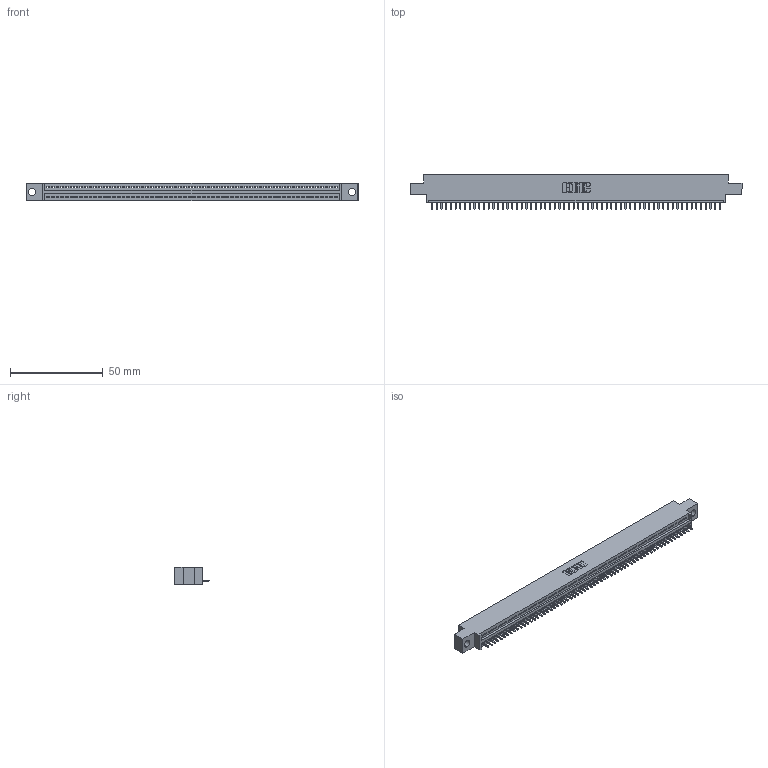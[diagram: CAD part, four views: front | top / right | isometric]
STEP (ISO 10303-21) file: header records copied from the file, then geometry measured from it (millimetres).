
FILE_DESCRIPTION (( 'STEP AP203' ), '1' );
FILE_NAME ('345-062-521-604.STEP', '2019-10-11T05:10:05', ( '' ), ( '' ), 'SwSTEP 2.0', 'SolidWorks 2016', '' );
FILE_SCHEMA (( 'CONFIG_CONTROL_DESIGN' ));
Length unit declared in the file: inch
Products named in the file (3): 345-062-521-604; 345-292-001_345-293-121; 345 Part_0.170 Offset - 0.156 Dia-TH
Assembly tree (63 placements, depth 2):
  345-062-521-604
    345 Part_0.170 Offset - 0.156 Dia-TH
    345-292-001_345-293-121  x62
Bounding box: 178.69 x 18.72 x 9.4 mm (x, y, z)
Volume: 16758.3 mm3; surface area: 21787.4 mm2
Topology: 63 solids, 63 shells, 3726 faces, 11265 edges, 7426 vertices
Faces by surface type: plane 2564, cylinder 1162
Entity records: 44123 total; most frequent: CARTESIAN_POINT 7650, ORIENTED_EDGE 7646, DIRECTION 6651, EDGE_CURVE 3823, VECTOR 3443, LINE 3443, VERTEX_POINT 2546, AXIS2_PLACEMENT_3D 1604
